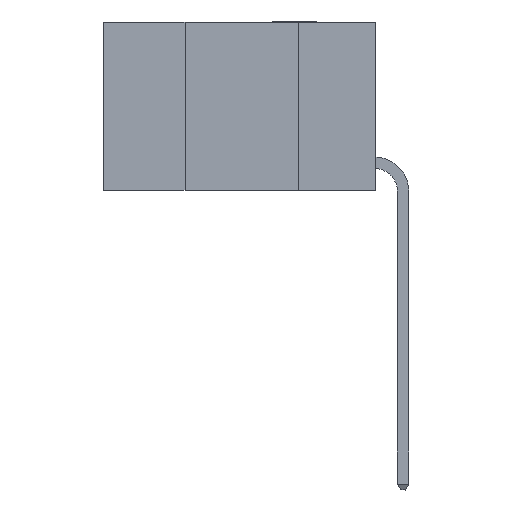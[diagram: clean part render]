
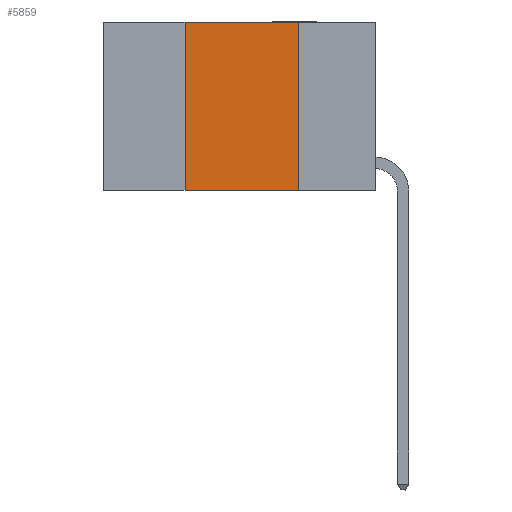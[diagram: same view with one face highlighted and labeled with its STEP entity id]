
A CAD part, left-side view. The second image highlights one B-rep face of the part: STEP entity #5859.
In plain terms, the highlighted planar face has unit normal (-1, 0, 0).
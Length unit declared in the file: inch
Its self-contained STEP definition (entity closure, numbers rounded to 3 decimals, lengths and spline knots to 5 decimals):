
#1115 = CARTESIAN_POINT ( 'NONE',  ( 0., 0.42, 0. ) ) ;
#1170 = ORIENTED_EDGE ( 'NONE', *, *, #4611, .F. ) ;
#1578 = CARTESIAN_POINT ( 'NONE',  ( 0., 0.6, -0.37 ) ) ;
#1646 = PLANE ( 'NONE',  #7797 ) ;
#1846 = VERTEX_POINT ( 'NONE', #5699 ) ;
#2561 = EDGE_LOOP ( 'NONE', ( #1170, #7091, #4460, #8194 ) ) ;
#2614 = CARTESIAN_POINT ( 'NONE',  ( 0., 0.6, 0. ) ) ;
#2681 = CARTESIAN_POINT ( 'NONE',  ( 0., 0.17, 0. ) ) ;
#2799 = VECTOR ( 'NONE', #8693, 39.37008 ) ;
#3287 = LINE ( 'NONE', #5069, #5098 ) ;
#3732 = VECTOR ( 'NONE', #6481, 39.37008 ) ;
#3929 = LINE ( 'NONE', #1578, #7740 ) ;
#3969 = DIRECTION ( 'NONE',  ( 1., 0., 0. ) ) ;
#4460 = ORIENTED_EDGE ( 'NONE', *, *, #7616, .F. ) ;
#4611 = EDGE_CURVE ( 'NONE', #9402, #9041, #3287, .T. ) ;
#5069 = CARTESIAN_POINT ( 'NONE',  ( 0., 0.17, 0. ) ) ;
#5098 = VECTOR ( 'NONE', #5843, 39.37008 ) ;
#5149 = EDGE_CURVE ( 'NONE', #1846, #9402, #6886, .T. ) ;
#5206 = FACE_OUTER_BOUND ( 'NONE', #2561, .T. ) ;
#5221 = CARTESIAN_POINT ( 'NONE',  ( 0., 0.17, -0.37 ) ) ;
#5699 = CARTESIAN_POINT ( 'NONE',  ( 0., 0.42, 0. ) ) ;
#5843 = DIRECTION ( 'NONE',  ( 0., 0., -1. ) ) ;
#5859 = ADVANCED_FACE ( 'NONE', ( #5206 ), #1646, .F. ) ;
#6174 = DIRECTION ( 'NONE',  ( 0., -1., 0. ) ) ;
#6481 = DIRECTION ( 'NONE',  ( 0., 0., 1. ) ) ;
#6886 = LINE ( 'NONE', #2614, #2799 ) ;
#7085 = LINE ( 'NONE', #1115, #3732 ) ;
#7091 = ORIENTED_EDGE ( 'NONE', *, *, #5149, .F. ) ;
#7616 = EDGE_CURVE ( 'NONE', #8320, #1846, #7085, .T. ) ;
#7740 = VECTOR ( 'NONE', #6174, 39.37008 ) ;
#7797 = AXIS2_PLACEMENT_3D ( 'NONE', #8513, #3969, #9189 ) ;
#8194 = ORIENTED_EDGE ( 'NONE', *, *, #9213, .T. ) ;
#8320 = VERTEX_POINT ( 'NONE', #9525 ) ;
#8513 = CARTESIAN_POINT ( 'NONE',  ( 0., 0.6, 0. ) ) ;
#8693 = DIRECTION ( 'NONE',  ( 0., -1., 0. ) ) ;
#9041 = VERTEX_POINT ( 'NONE', #5221 ) ;
#9189 = DIRECTION ( 'NONE',  ( 0., 0., -1. ) ) ;
#9213 = EDGE_CURVE ( 'NONE', #8320, #9041, #3929, .T. ) ;
#9402 = VERTEX_POINT ( 'NONE', #2681 ) ;
#9525 = CARTESIAN_POINT ( 'NONE',  ( 0., 0.42, -0.37 ) ) ;
